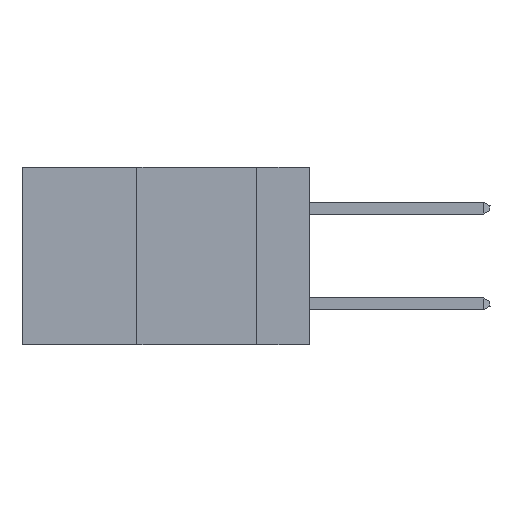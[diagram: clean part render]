
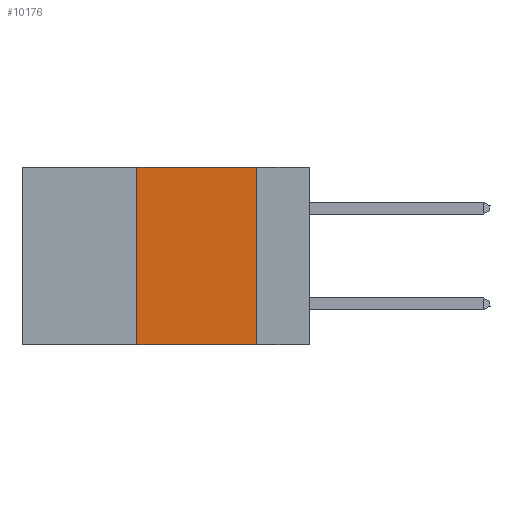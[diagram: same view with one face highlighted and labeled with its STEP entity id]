
A CAD part, left-side view. The second image highlights one B-rep face of the part: STEP entity #10176.
In plain terms, the highlighted planar face has unit normal (-1, 0, 0).
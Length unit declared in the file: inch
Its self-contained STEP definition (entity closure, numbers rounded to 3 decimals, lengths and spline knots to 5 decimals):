
#640 = VECTOR ( 'NONE', #9968, 39.37008 ) ;
#886 = ORIENTED_EDGE ( 'NONE', *, *, #14201, .T. ) ;
#933 = CARTESIAN_POINT ( 'NONE',  ( 0., 0.11, 0. ) ) ;
#1139 = DIRECTION ( 'NONE',  ( 1., 0., 0. ) ) ;
#1744 = CARTESIAN_POINT ( 'NONE',  ( 0., 0.6, -0.37 ) ) ;
#3015 = CARTESIAN_POINT ( 'NONE',  ( 0., 0.11, -0.37 ) ) ;
#3236 = DIRECTION ( 'NONE',  ( 0., 0., 1. ) ) ;
#3968 = VECTOR ( 'NONE', #21161, 39.37008 ) ;
#6027 = DIRECTION ( 'NONE',  ( 0., -1., 0. ) ) ;
#6318 = CARTESIAN_POINT ( 'NONE',  ( 0., 0.36, 0. ) ) ;
#6639 = EDGE_CURVE ( 'NONE', #16110, #22388, #8016, .T. ) ;
#7123 = VERTEX_POINT ( 'NONE', #21916 ) ;
#7440 = ORIENTED_EDGE ( 'NONE', *, *, #6639, .F. ) ;
#7736 = PLANE ( 'NONE',  #13262 ) ;
#8016 = LINE ( 'NONE', #21426, #640 ) ;
#8995 = LINE ( 'NONE', #9393, #3968 ) ;
#9219 = DIRECTION ( 'NONE',  ( 0., 0., -1. ) ) ;
#9393 = CARTESIAN_POINT ( 'NONE',  ( 0., 0.11, 0. ) ) ;
#9968 = DIRECTION ( 'NONE',  ( 0., -1., 0. ) ) ;
#10176 = ADVANCED_FACE ( 'NONE', ( #14051 ), #7736, .F. ) ;
#13094 = CARTESIAN_POINT ( 'NONE',  ( 0., 0.36, 0. ) ) ;
#13262 = AXIS2_PLACEMENT_3D ( 'NONE', #15907, #1139, #9219 ) ;
#13830 = LINE ( 'NONE', #1744, #18595 ) ;
#14043 = VECTOR ( 'NONE', #3236, 39.37008 ) ;
#14051 = FACE_OUTER_BOUND ( 'NONE', #18628, .T. ) ;
#14201 = EDGE_CURVE ( 'NONE', #7123, #17541, #13830, .T. ) ;
#15907 = CARTESIAN_POINT ( 'NONE',  ( 0., 0.6, 0. ) ) ;
#16110 = VERTEX_POINT ( 'NONE', #13094 ) ;
#17118 = EDGE_CURVE ( 'NONE', #22388, #17541, #8995, .T. ) ;
#17541 = VERTEX_POINT ( 'NONE', #3015 ) ;
#18283 = EDGE_CURVE ( 'NONE', #7123, #16110, #22622, .T. ) ;
#18595 = VECTOR ( 'NONE', #6027, 39.37008 ) ;
#18628 = EDGE_LOOP ( 'NONE', ( #18859, #7440, #23832, #886 ) ) ;
#18859 = ORIENTED_EDGE ( 'NONE', *, *, #17118, .F. ) ;
#21161 = DIRECTION ( 'NONE',  ( 0., 0., -1. ) ) ;
#21426 = CARTESIAN_POINT ( 'NONE',  ( 0., 0.6, 0. ) ) ;
#21916 = CARTESIAN_POINT ( 'NONE',  ( 0., 0.36, -0.37 ) ) ;
#22388 = VERTEX_POINT ( 'NONE', #933 ) ;
#22622 = LINE ( 'NONE', #6318, #14043 ) ;
#23832 = ORIENTED_EDGE ( 'NONE', *, *, #18283, .F. ) ;
